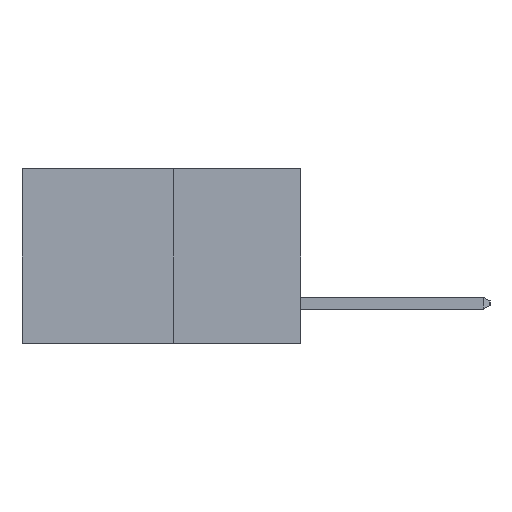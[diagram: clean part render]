
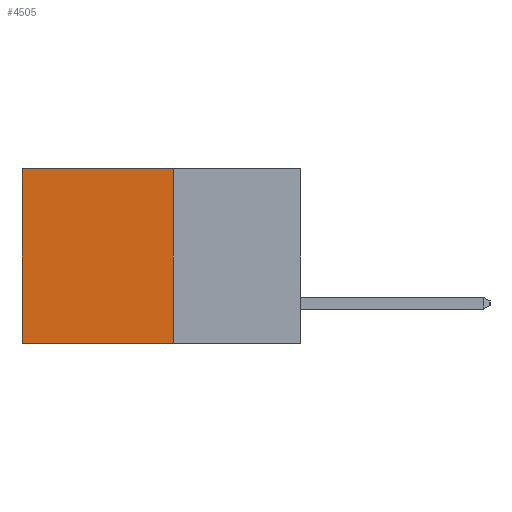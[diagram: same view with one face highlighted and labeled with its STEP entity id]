
A CAD part, left-side view. The second image highlights one B-rep face of the part: STEP entity #4505.
In plain terms, the highlighted planar face has unit normal (-1, 0, 0).
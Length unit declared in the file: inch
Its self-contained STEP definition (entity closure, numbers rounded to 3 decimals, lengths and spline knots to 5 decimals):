
#849 = CARTESIAN_POINT ( 'NONE',  ( 0.277, 0.27, 0. ) ) ;
#2196 = DIRECTION ( 'NONE',  ( 0., 0., -1. ) ) ;
#2453 = EDGE_LOOP ( 'NONE', ( #17346, #18559, #19763, #20974 ) ) ;
#2869 = CARTESIAN_POINT ( 'NONE',  ( 0.277, 0.27, -0.37 ) ) ;
#2965 = VECTOR ( 'NONE', #2196, 39.37008 ) ;
#3444 = EDGE_CURVE ( 'NONE', #21181, #19253, #10411, .T. ) ;
#4195 = CARTESIAN_POINT ( 'NONE',  ( 0.277, 0.59, -0.37 ) ) ;
#4505 = ADVANCED_FACE ( 'NONE', ( #16285 ), #20826, .F. ) ;
#4520 = DIRECTION ( 'NONE',  ( 0., 0., -1. ) ) ;
#5828 = CARTESIAN_POINT ( 'NONE',  ( 0.277, 0.27, -0.37 ) ) ;
#7894 = VERTEX_POINT ( 'NONE', #11696 ) ;
#8655 = DIRECTION ( 'NONE',  ( 1., 0., 0. ) ) ;
#9305 = CARTESIAN_POINT ( 'NONE',  ( 0.277, 0.27, -0.37 ) ) ;
#10265 = EDGE_CURVE ( 'NONE', #14070, #7894, #21384, .T. ) ;
#10411 = LINE ( 'NONE', #2869, #24997 ) ;
#10575 = LINE ( 'NONE', #4195, #19515 ) ;
#10699 = DIRECTION ( 'NONE',  ( 0., 1., 0. ) ) ;
#11558 = EDGE_CURVE ( 'NONE', #7894, #19253, #10575, .T. ) ;
#11696 = CARTESIAN_POINT ( 'NONE',  ( 0.277, 0.59, 0. ) ) ;
#13324 = LINE ( 'NONE', #19549, #2965 ) ;
#13749 = DIRECTION ( 'NONE',  ( 0., 1., 0. ) ) ;
#14070 = VERTEX_POINT ( 'NONE', #849 ) ;
#14077 = AXIS2_PLACEMENT_3D ( 'NONE', #9305, #8655, #4520 ) ;
#16285 = FACE_OUTER_BOUND ( 'NONE', #2453, .T. ) ;
#16883 = VECTOR ( 'NONE', #13749, 39.37008 ) ;
#17346 = ORIENTED_EDGE ( 'NONE', *, *, #11558, .T. ) ;
#18559 = ORIENTED_EDGE ( 'NONE', *, *, #3444, .F. ) ;
#18951 = CARTESIAN_POINT ( 'NONE',  ( 0.277, 0.59, -0.37 ) ) ;
#19253 = VERTEX_POINT ( 'NONE', #18951 ) ;
#19515 = VECTOR ( 'NONE', #21555, 39.37008 ) ;
#19549 = CARTESIAN_POINT ( 'NONE',  ( 0.277, 0.27, -0.37 ) ) ;
#19763 = ORIENTED_EDGE ( 'NONE', *, *, #23953, .F. ) ;
#20826 = PLANE ( 'NONE',  #14077 ) ;
#20974 = ORIENTED_EDGE ( 'NONE', *, *, #10265, .T. ) ;
#21181 = VERTEX_POINT ( 'NONE', #5828 ) ;
#21384 = LINE ( 'NONE', #23262, #16883 ) ;
#21555 = DIRECTION ( 'NONE',  ( 0., 0., -1. ) ) ;
#23262 = CARTESIAN_POINT ( 'NONE',  ( 0.277, 0.27, 0. ) ) ;
#23953 = EDGE_CURVE ( 'NONE', #14070, #21181, #13324, .T. ) ;
#24997 = VECTOR ( 'NONE', #10699, 39.37008 ) ;
